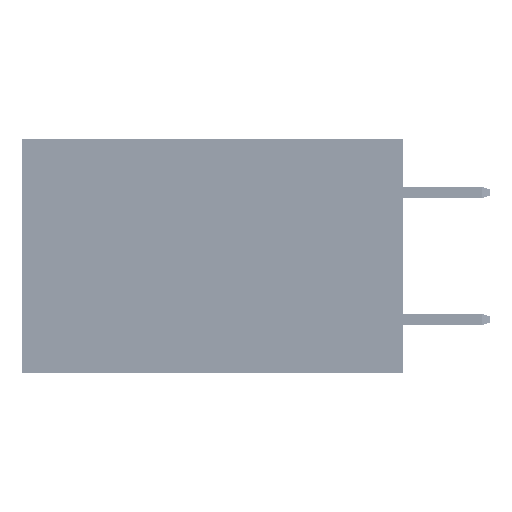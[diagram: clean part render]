
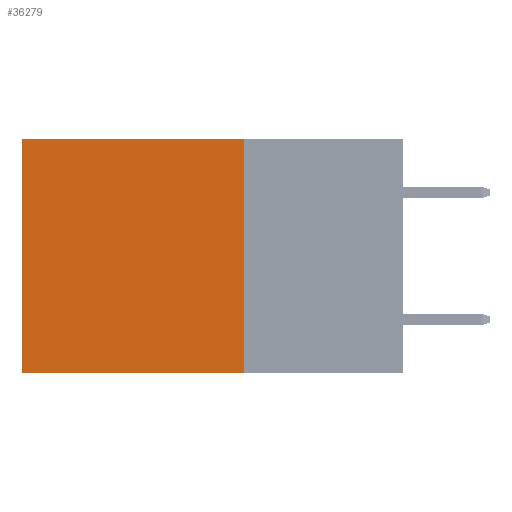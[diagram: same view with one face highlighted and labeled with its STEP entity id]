
A CAD part, left-side view. The second image highlights one B-rep face of the part: STEP entity #36279.
In plain terms, the highlighted planar face has unit normal (-1, 0, 0).
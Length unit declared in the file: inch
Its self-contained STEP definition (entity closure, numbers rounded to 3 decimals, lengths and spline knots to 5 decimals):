
#495 = FACE_OUTER_BOUND ( 'NONE', #34751, .T. ) ;
#1818 = LINE ( 'NONE', #9836, #13401 ) ;
#2803 = VECTOR ( 'NONE', #33201, 39.37008 ) ;
#3530 = CARTESIAN_POINT ( 'NONE',  ( 0.2875, 0.6, 0. ) ) ;
#4254 = EDGE_CURVE ( 'NONE', #9456, #46525, #7178, .T. ) ;
#4403 = CARTESIAN_POINT ( 'NONE',  ( 0.2875, 0.25, 0. ) ) ;
#5185 = ORIENTED_EDGE ( 'NONE', *, *, #7270, .F. ) ;
#7178 = LINE ( 'NONE', #3530, #2803 ) ;
#7270 = EDGE_CURVE ( 'NONE', #36900, #46525, #31365, .T. ) ;
#9456 = VERTEX_POINT ( 'NONE', #23260 ) ;
#9802 = EDGE_CURVE ( 'NONE', #33568, #36900, #21752, .T. ) ;
#9836 = CARTESIAN_POINT ( 'NONE',  ( 0.2875, 0.25, 0. ) ) ;
#11501 = DIRECTION ( 'NONE',  ( 0., 0., -1. ) ) ;
#13401 = VECTOR ( 'NONE', #27842, 39.37008 ) ;
#14827 = CARTESIAN_POINT ( 'NONE',  ( 0.2875, 0.6, -0.37 ) ) ;
#15310 = ORIENTED_EDGE ( 'NONE', *, *, #9802, .F. ) ;
#16078 = DIRECTION ( 'NONE',  ( 0., 0., -1. ) ) ;
#20883 = CARTESIAN_POINT ( 'NONE',  ( 0.2875, 0.25, -0.37 ) ) ;
#21752 = LINE ( 'NONE', #40679, #44205 ) ;
#23260 = CARTESIAN_POINT ( 'NONE',  ( 0.2875, 0.6, 0. ) ) ;
#23382 = DIRECTION ( 'NONE',  ( 1., 0., 0. ) ) ;
#23568 = CARTESIAN_POINT ( 'NONE',  ( 0.2875, 0.25, 0. ) ) ;
#24078 = DIRECTION ( 'NONE',  ( 0., 1., 0. ) ) ;
#25558 = ORIENTED_EDGE ( 'NONE', *, *, #27420, .T. ) ;
#27420 = EDGE_CURVE ( 'NONE', #33568, #9456, #1818, .T. ) ;
#27713 = CARTESIAN_POINT ( 'NONE',  ( 0.2875, 0.25, -0.37 ) ) ;
#27842 = DIRECTION ( 'NONE',  ( 0., 1., 0. ) ) ;
#31365 = LINE ( 'NONE', #27713, #37859 ) ;
#32952 = AXIS2_PLACEMENT_3D ( 'NONE', #4403, #23382, #16078 ) ;
#33201 = DIRECTION ( 'NONE',  ( 0., 0., -1. ) ) ;
#33568 = VERTEX_POINT ( 'NONE', #23568 ) ;
#34751 = EDGE_LOOP ( 'NONE', ( #39701, #5185, #15310, #25558 ) ) ;
#36279 = ADVANCED_FACE ( 'NONE', ( #495 ), #42075, .F. ) ;
#36900 = VERTEX_POINT ( 'NONE', #20883 ) ;
#37859 = VECTOR ( 'NONE', #24078, 39.37008 ) ;
#39701 = ORIENTED_EDGE ( 'NONE', *, *, #4254, .T. ) ;
#40679 = CARTESIAN_POINT ( 'NONE',  ( 0.2875, 0.25, 0. ) ) ;
#42075 = PLANE ( 'NONE',  #32952 ) ;
#44205 = VECTOR ( 'NONE', #11501, 39.37008 ) ;
#46525 = VERTEX_POINT ( 'NONE', #14827 ) ;
